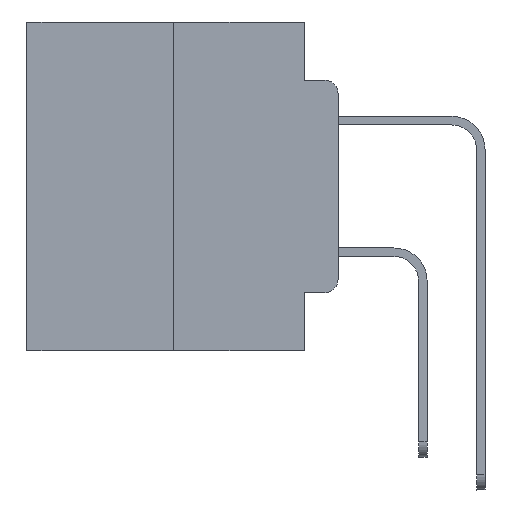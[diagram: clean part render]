
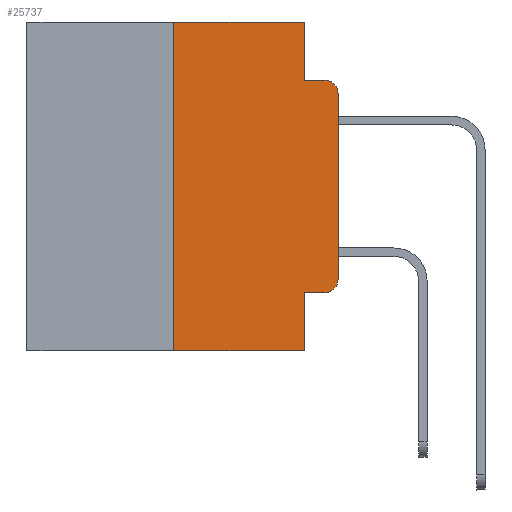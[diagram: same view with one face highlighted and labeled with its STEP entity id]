
A CAD part, left-side view. The second image highlights one B-rep face of the part: STEP entity #25737.
In plain terms, the highlighted planar face has unit normal (-1, 0, 0).
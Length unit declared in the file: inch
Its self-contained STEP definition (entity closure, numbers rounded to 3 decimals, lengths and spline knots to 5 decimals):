
#6 = EDGE_CURVE ( 'NONE', #27492, #3603, #16654, .T. ) ;
#953 = CARTESIAN_POINT ( 'NONE',  ( 0., 0.473, 0. ) ) ;
#1532 = CARTESIAN_POINT ( 'NONE',  ( 0., 0.051, -0.0885 ) ) ;
#1992 = VECTOR ( 'NONE', #18563, 39.37008 ) ;
#2774 = EDGE_CURVE ( 'NONE', #26407, #3753, #9900, .T. ) ;
#3178 = LINE ( 'NONE', #15796, #6870 ) ;
#3217 = CARTESIAN_POINT ( 'NONE',  ( 0., 0.25, 0. ) ) ;
#3302 = VECTOR ( 'NONE', #3830, 39.37008 ) ;
#3603 = VERTEX_POINT ( 'NONE', #23596 ) ;
#3753 = VERTEX_POINT ( 'NONE', #8941 ) ;
#3830 = DIRECTION ( 'NONE',  ( 0., -1., 0. ) ) ;
#4642 = ORIENTED_EDGE ( 'NONE', *, *, #12986, .T. ) ;
#4678 = VERTEX_POINT ( 'NONE', #12996 ) ;
#4864 = DIRECTION ( 'NONE',  ( 0., 0., -1. ) ) ;
#4884 = ORIENTED_EDGE ( 'NONE', *, *, #5246, .F. ) ;
#5246 = EDGE_CURVE ( 'NONE', #17337, #26407, #17508, .T. ) ;
#5765 = ORIENTED_EDGE ( 'NONE', *, *, #6, .F. ) ;
#5789 = VECTOR ( 'NONE', #8579, 39.37008 ) ;
#6243 = CARTESIAN_POINT ( 'NONE',  ( 0., 0.02, -0.1085 ) ) ;
#6537 = ORIENTED_EDGE ( 'NONE', *, *, #24519, .T. ) ;
#6870 = VECTOR ( 'NONE', #11690, 39.37008 ) ;
#7215 = EDGE_CURVE ( 'NONE', #13805, #3753, #26321, .T. ) ;
#7727 = VERTEX_POINT ( 'NONE', #22242 ) ;
#7941 = CARTESIAN_POINT ( 'NONE',  ( 0., 0., 0. ) ) ;
#8154 = DIRECTION ( 'NONE',  ( 0., 0., -1. ) ) ;
#8459 = AXIS2_PLACEMENT_3D ( 'NONE', #953, #9605, #25273 ) ;
#8579 = DIRECTION ( 'NONE',  ( 0., 0., -1. ) ) ;
#8941 = CARTESIAN_POINT ( 'NONE',  ( 0., 0.02, -0.0885 ) ) ;
#9369 = EDGE_CURVE ( 'NONE', #7727, #3603, #3178, .T. ) ;
#9605 = DIRECTION ( 'NONE',  ( 1., 0., 0. ) ) ;
#9796 = ORIENTED_EDGE ( 'NONE', *, *, #13917, .F. ) ;
#9900 = LINE ( 'NONE', #1532, #23463 ) ;
#10172 = PLANE ( 'NONE',  #8459 ) ;
#10184 = DIRECTION ( 'NONE',  ( 0., -1., 0. ) ) ;
#10661 = ORIENTED_EDGE ( 'NONE', *, *, #9369, .T. ) ;
#10775 = DIRECTION ( 'NONE',  ( -1., 0., 0. ) ) ;
#11690 = DIRECTION ( 'NONE',  ( 0., -1., 0. ) ) ;
#11754 = AXIS2_PLACEMENT_3D ( 'NONE', #6243, #10775, #4864 ) ;
#11866 = FACE_OUTER_BOUND ( 'NONE', #24598, .T. ) ;
#11978 = VECTOR ( 'NONE', #19826, 39.37008 ) ;
#12194 = LINE ( 'NONE', #7941, #1992 ) ;
#12289 = VERTEX_POINT ( 'NONE', #26077 ) ;
#12862 = CARTESIAN_POINT ( 'NONE',  ( 0., 0.051, -0.4115 ) ) ;
#12863 = DIRECTION ( 'NONE',  ( -1., 0., 0. ) ) ;
#12875 = CARTESIAN_POINT ( 'NONE',  ( 0., 0.051, 0. ) ) ;
#12986 = EDGE_CURVE ( 'NONE', #4678, #13805, #12194, .T. ) ;
#12996 = CARTESIAN_POINT ( 'NONE',  ( 0., 0., -0.3915 ) ) ;
#13501 = EDGE_CURVE ( 'NONE', #12289, #17337, #20036, .T. ) ;
#13564 = ORIENTED_EDGE ( 'NONE', *, *, #2774, .F. ) ;
#13805 = VERTEX_POINT ( 'NONE', #14625 ) ;
#13820 = CIRCLE ( 'NONE', #26995, 0.02 ) ;
#13917 = EDGE_CURVE ( 'NONE', #7727, #12289, #15828, .T. ) ;
#14625 = CARTESIAN_POINT ( 'NONE',  ( 0., 0., -0.1085 ) ) ;
#15796 = CARTESIAN_POINT ( 'NONE',  ( 0., 0.473, -0.5 ) ) ;
#15828 = LINE ( 'NONE', #3217, #11978 ) ;
#16496 = CARTESIAN_POINT ( 'NONE',  ( 0., 0.02, -0.4115 ) ) ;
#16654 = LINE ( 'NONE', #27643, #27865 ) ;
#17088 = CARTESIAN_POINT ( 'NONE',  ( 0., 0.051, 0. ) ) ;
#17209 = ORIENTED_EDGE ( 'NONE', *, *, #7215, .T. ) ;
#17337 = VERTEX_POINT ( 'NONE', #12875 ) ;
#17508 = LINE ( 'NONE', #17088, #5789 ) ;
#18563 = DIRECTION ( 'NONE',  ( 0., 0., 1. ) ) ;
#18701 = CARTESIAN_POINT ( 'NONE',  ( 0., 0.051, -0.4115 ) ) ;
#19239 = DIRECTION ( 'NONE',  ( 0., 0., -1. ) ) ;
#19826 = DIRECTION ( 'NONE',  ( 0., 0., 1. ) ) ;
#20036 = LINE ( 'NONE', #26476, #20570 ) ;
#20175 = DIRECTION ( 'NONE',  ( 0., -1., 0. ) ) ;
#20570 = VECTOR ( 'NONE', #20175, 39.37008 ) ;
#21516 = EDGE_CURVE ( 'NONE', #27492, #26566, #23136, .T. ) ;
#22242 = CARTESIAN_POINT ( 'NONE',  ( 0., 0.25, -0.5 ) ) ;
#23136 = LINE ( 'NONE', #18701, #3302 ) ;
#23463 = VECTOR ( 'NONE', #10184, 39.37008 ) ;
#23539 = CARTESIAN_POINT ( 'NONE',  ( 0., 0.02, -0.3915 ) ) ;
#23596 = CARTESIAN_POINT ( 'NONE',  ( 0., 0.051, -0.5 ) ) ;
#24519 = EDGE_CURVE ( 'NONE', #26566, #4678, #13820, .T. ) ;
#24598 = EDGE_LOOP ( 'NONE', ( #4642, #17209, #13564, #4884, #27013, #9796, #10661, #5765, #27593, #6537 ) ) ;
#25273 = DIRECTION ( 'NONE',  ( 0., 0., -1. ) ) ;
#25737 = ADVANCED_FACE ( 'NONE', ( #11866 ), #10172, .F. ) ;
#26077 = CARTESIAN_POINT ( 'NONE',  ( 0., 0.25, 0. ) ) ;
#26321 = CIRCLE ( 'NONE', #11754, 0.02 ) ;
#26407 = VERTEX_POINT ( 'NONE', #26642 ) ;
#26476 = CARTESIAN_POINT ( 'NONE',  ( 0., 0.473, 0. ) ) ;
#26566 = VERTEX_POINT ( 'NONE', #16496 ) ;
#26642 = CARTESIAN_POINT ( 'NONE',  ( 0., 0.051, -0.0885 ) ) ;
#26995 = AXIS2_PLACEMENT_3D ( 'NONE', #23539, #12863, #19239 ) ;
#27013 = ORIENTED_EDGE ( 'NONE', *, *, #13501, .F. ) ;
#27492 = VERTEX_POINT ( 'NONE', #12862 ) ;
#27593 = ORIENTED_EDGE ( 'NONE', *, *, #21516, .T. ) ;
#27643 = CARTESIAN_POINT ( 'NONE',  ( 0., 0.051, 0. ) ) ;
#27865 = VECTOR ( 'NONE', #8154, 39.37008 ) ;
